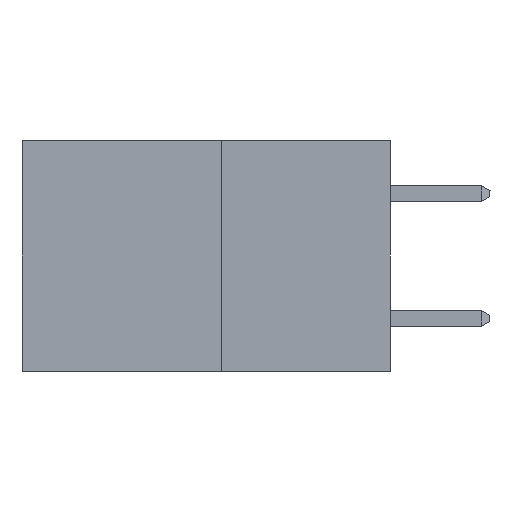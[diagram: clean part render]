
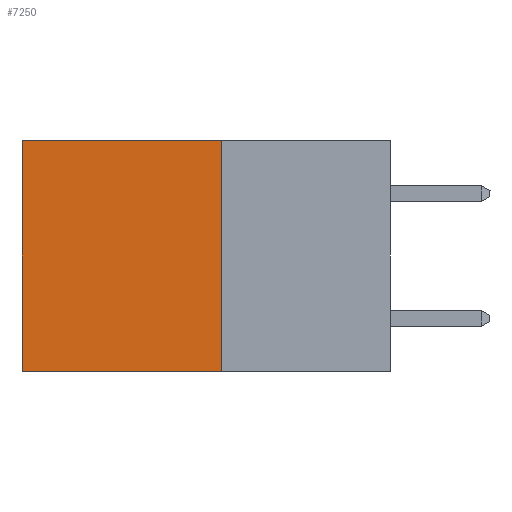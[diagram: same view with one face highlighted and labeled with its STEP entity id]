
A CAD part, left-side view. The second image highlights one B-rep face of the part: STEP entity #7250.
In plain terms, the highlighted planar face has unit normal (-1, 0, 0).
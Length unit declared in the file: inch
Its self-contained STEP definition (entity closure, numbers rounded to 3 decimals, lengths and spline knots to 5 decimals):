
#11 = AXIS2_PLACEMENT_3D ( 'NONE', #370, #6527, #1285 ) ;
#85 = DIRECTION ( 'NONE',  ( 0., 0., -1. ) ) ;
#107 = LINE ( 'NONE', #10420, #9066 ) ;
#370 = CARTESIAN_POINT ( 'NONE',  ( 0.277, 0.27, -0.37 ) ) ;
#566 = CARTESIAN_POINT ( 'NONE',  ( 0.277, 0.27, -0.37 ) ) ;
#825 = EDGE_LOOP ( 'NONE', ( #7867, #7945, #6690, #10427 ) ) ;
#1065 = VERTEX_POINT ( 'NONE', #10677 ) ;
#1093 = VECTOR ( 'NONE', #85, 39.37008 ) ;
#1285 = DIRECTION ( 'NONE',  ( 0., 0., -1. ) ) ;
#1526 = DIRECTION ( 'NONE',  ( 0., 1., 0. ) ) ;
#1566 = CARTESIAN_POINT ( 'NONE',  ( 0.277, 0.27, -0.37 ) ) ;
#1635 = VERTEX_POINT ( 'NONE', #4899 ) ;
#1809 = CARTESIAN_POINT ( 'NONE',  ( 0.277, 0.27, 0. ) ) ;
#2342 = VERTEX_POINT ( 'NONE', #10140 ) ;
#2679 = DIRECTION ( 'NONE',  ( 0., 1., 0. ) ) ;
#3460 = LINE ( 'NONE', #10354, #1093 ) ;
#4862 = VECTOR ( 'NONE', #2679, 39.37008 ) ;
#4899 = CARTESIAN_POINT ( 'NONE',  ( 0.277, 0.59, -0.37 ) ) ;
#5406 = LINE ( 'NONE', #1809, #4862 ) ;
#5494 = VECTOR ( 'NONE', #1526, 39.37008 ) ;
#5746 = LINE ( 'NONE', #1566, #5494 ) ;
#6230 = DIRECTION ( 'NONE',  ( 0., 0., -1. ) ) ;
#6313 = EDGE_CURVE ( 'NONE', #1065, #9035, #3460, .T. ) ;
#6527 = DIRECTION ( 'NONE',  ( 1., 0., 0. ) ) ;
#6690 = ORIENTED_EDGE ( 'NONE', *, *, #6313, .F. ) ;
#7250 = ADVANCED_FACE ( 'NONE', ( #10298 ), #9869, .F. ) ;
#7867 = ORIENTED_EDGE ( 'NONE', *, *, #10347, .T. ) ;
#7945 = ORIENTED_EDGE ( 'NONE', *, *, #10974, .F. ) ;
#9035 = VERTEX_POINT ( 'NONE', #566 ) ;
#9066 = VECTOR ( 'NONE', #6230, 39.37008 ) ;
#9136 = EDGE_CURVE ( 'NONE', #1065, #2342, #5406, .T. ) ;
#9869 = PLANE ( 'NONE',  #11 ) ;
#10140 = CARTESIAN_POINT ( 'NONE',  ( 0.277, 0.59, 0. ) ) ;
#10298 = FACE_OUTER_BOUND ( 'NONE', #825, .T. ) ;
#10347 = EDGE_CURVE ( 'NONE', #2342, #1635, #107, .T. ) ;
#10354 = CARTESIAN_POINT ( 'NONE',  ( 0.277, 0.27, -0.37 ) ) ;
#10420 = CARTESIAN_POINT ( 'NONE',  ( 0.277, 0.59, -0.37 ) ) ;
#10427 = ORIENTED_EDGE ( 'NONE', *, *, #9136, .T. ) ;
#10677 = CARTESIAN_POINT ( 'NONE',  ( 0.277, 0.27, 0. ) ) ;
#10974 = EDGE_CURVE ( 'NONE', #9035, #1635, #5746, .T. ) ;
